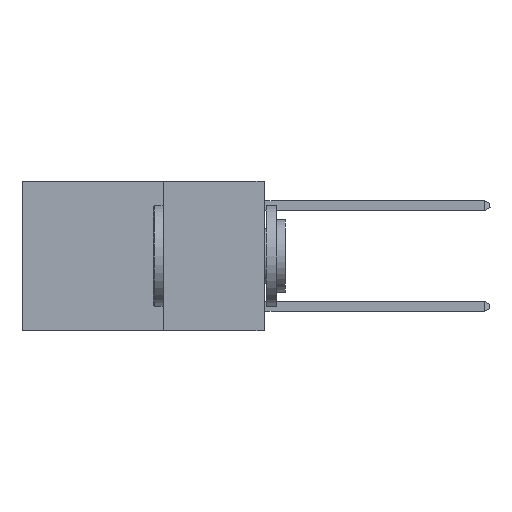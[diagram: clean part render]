
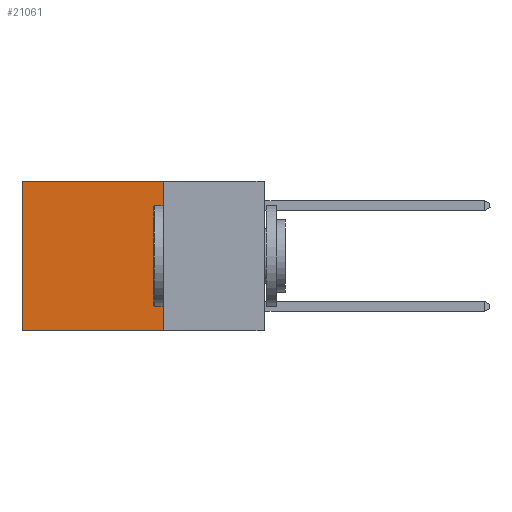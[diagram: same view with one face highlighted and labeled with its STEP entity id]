
A CAD part, left-side view. The second image highlights one B-rep face of the part: STEP entity #21061.
In plain terms, the highlighted planar face has unit normal (-1, 0, 0).
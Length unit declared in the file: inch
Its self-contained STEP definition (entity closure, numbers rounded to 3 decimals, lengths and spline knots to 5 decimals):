
#175 = EDGE_CURVE ( 'NONE', #7440, #20487, #12392, .T. ) ;
#1627 = EDGE_LOOP ( 'NONE', ( #5098, #15483, #22469, #20981 ) ) ;
#3224 = EDGE_CURVE ( 'NONE', #16400, #20487, #17728, .T. ) ;
#4449 = DIRECTION ( 'NONE',  ( 0., 0., -1. ) ) ;
#5098 = ORIENTED_EDGE ( 'NONE', *, *, #175, .T. ) ;
#5706 = CARTESIAN_POINT ( 'NONE',  ( 0.2625, 0.25, -0.37 ) ) ;
#6317 = DIRECTION ( 'NONE',  ( 1., 0., 0. ) ) ;
#6621 = CARTESIAN_POINT ( 'NONE',  ( 0.2625, 0.25, 0. ) ) ;
#7440 = VERTEX_POINT ( 'NONE', #11238 ) ;
#7733 = DIRECTION ( 'NONE',  ( 0., 1., 0. ) ) ;
#8099 = VECTOR ( 'NONE', #22023, 39.37008 ) ;
#9312 = LINE ( 'NONE', #6621, #8099 ) ;
#9614 = EDGE_CURVE ( 'NONE', #24893, #16400, #9312, .T. ) ;
#10101 = VECTOR ( 'NONE', #7733, 39.37008 ) ;
#11238 = CARTESIAN_POINT ( 'NONE',  ( 0.2625, 0.6, 0. ) ) ;
#11820 = AXIS2_PLACEMENT_3D ( 'NONE', #14020, #6317, #4449 ) ;
#12392 = LINE ( 'NONE', #15770, #15731 ) ;
#12394 = CARTESIAN_POINT ( 'NONE',  ( 0.2625, 0.25, -0.37 ) ) ;
#12616 = VECTOR ( 'NONE', #17639, 39.37008 ) ;
#13694 = PLANE ( 'NONE',  #11820 ) ;
#14020 = CARTESIAN_POINT ( 'NONE',  ( 0.2625, 0.25, 0. ) ) ;
#15483 = ORIENTED_EDGE ( 'NONE', *, *, #3224, .F. ) ;
#15731 = VECTOR ( 'NONE', #19651, 39.37008 ) ;
#15770 = CARTESIAN_POINT ( 'NONE',  ( 0.2625, 0.6, 0. ) ) ;
#16400 = VERTEX_POINT ( 'NONE', #12394 ) ;
#17608 = EDGE_CURVE ( 'NONE', #24893, #7440, #24348, .T. ) ;
#17639 = DIRECTION ( 'NONE',  ( 0., 1., 0. ) ) ;
#17728 = LINE ( 'NONE', #5706, #10101 ) ;
#17826 = FACE_OUTER_BOUND ( 'NONE', #1627, .T. ) ;
#19321 = CARTESIAN_POINT ( 'NONE',  ( 0.2625, 0.25, 0. ) ) ;
#19651 = DIRECTION ( 'NONE',  ( 0., 0., -1. ) ) ;
#19719 = CARTESIAN_POINT ( 'NONE',  ( 0.2625, 0.6, -0.37 ) ) ;
#20487 = VERTEX_POINT ( 'NONE', #19719 ) ;
#20981 = ORIENTED_EDGE ( 'NONE', *, *, #17608, .T. ) ;
#21061 = ADVANCED_FACE ( 'NONE', ( #17826 ), #13694, .F. ) ;
#22023 = DIRECTION ( 'NONE',  ( 0., 0., -1. ) ) ;
#22469 = ORIENTED_EDGE ( 'NONE', *, *, #9614, .F. ) ;
#24335 = CARTESIAN_POINT ( 'NONE',  ( 0.2625, 0.25, 0. ) ) ;
#24348 = LINE ( 'NONE', #19321, #12616 ) ;
#24893 = VERTEX_POINT ( 'NONE', #24335 ) ;
